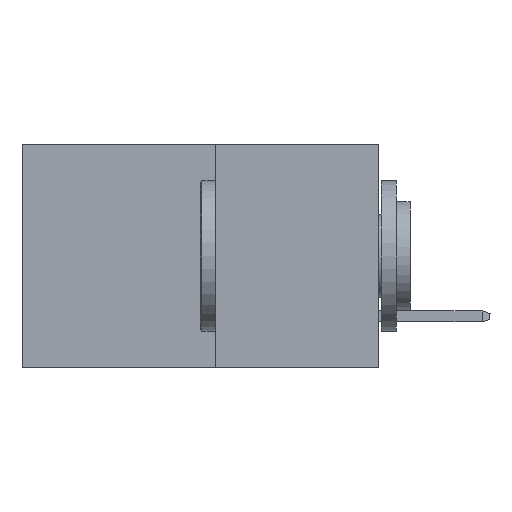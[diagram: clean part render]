
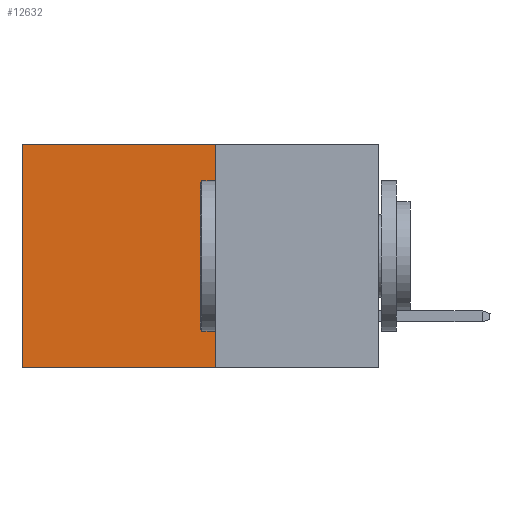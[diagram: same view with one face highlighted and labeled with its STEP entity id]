
A CAD part, left-side view. The second image highlights one B-rep face of the part: STEP entity #12632.
In plain terms, the highlighted planar face has unit normal (-1, 0, 0).
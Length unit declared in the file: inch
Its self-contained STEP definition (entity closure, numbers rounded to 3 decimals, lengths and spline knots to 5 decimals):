
#191 = EDGE_CURVE ( 'NONE', #2606, #7207, #2613, .T. ) ;
#749 = VECTOR ( 'NONE', #18762, 39.37008 ) ;
#1386 = ORIENTED_EDGE ( 'NONE', *, *, #4446, .T. ) ;
#1674 = VERTEX_POINT ( 'NONE', #5386 ) ;
#2606 = VERTEX_POINT ( 'NONE', #9807 ) ;
#2611 = CARTESIAN_POINT ( 'NONE',  ( 0.277, 0.27, 0. ) ) ;
#2613 = LINE ( 'NONE', #2611, #6604 ) ;
#3607 = ORIENTED_EDGE ( 'NONE', *, *, #17054, .F. ) ;
#4293 = PLANE ( 'NONE',  #8419 ) ;
#4446 = EDGE_CURVE ( 'NONE', #7207, #8948, #5085, .T. ) ;
#4540 = VECTOR ( 'NONE', #20747, 39.37008 ) ;
#5085 = LINE ( 'NONE', #20797, #4540 ) ;
#5386 = CARTESIAN_POINT ( 'NONE',  ( 0.277, 0.27, -0.37 ) ) ;
#5595 = CARTESIAN_POINT ( 'NONE',  ( 0.277, 0.27, -0.37 ) ) ;
#6604 = VECTOR ( 'NONE', #13789, 39.37008 ) ;
#7207 = VERTEX_POINT ( 'NONE', #15100 ) ;
#7413 = ORIENTED_EDGE ( 'NONE', *, *, #19953, .F. ) ;
#7571 = CARTESIAN_POINT ( 'NONE',  ( 0.277, 0.27, -0.37 ) ) ;
#7633 = FACE_OUTER_BOUND ( 'NONE', #19626, .T. ) ;
#7637 = DIRECTION ( 'NONE',  ( 0., 0., -1. ) ) ;
#8419 = AXIS2_PLACEMENT_3D ( 'NONE', #7571, #17523, #7637 ) ;
#8663 = VECTOR ( 'NONE', #21054, 39.37008 ) ;
#8948 = VERTEX_POINT ( 'NONE', #12015 ) ;
#9196 = LINE ( 'NONE', #19438, #8663 ) ;
#9677 = LINE ( 'NONE', #5595, #749 ) ;
#9807 = CARTESIAN_POINT ( 'NONE',  ( 0.277, 0.27, 0. ) ) ;
#12015 = CARTESIAN_POINT ( 'NONE',  ( 0.277, 0.59, -0.37 ) ) ;
#12632 = ADVANCED_FACE ( 'NONE', ( #7633 ), #4293, .F. ) ;
#13789 = DIRECTION ( 'NONE',  ( 0., 1., 0. ) ) ;
#15100 = CARTESIAN_POINT ( 'NONE',  ( 0.277, 0.59, 0. ) ) ;
#15321 = ORIENTED_EDGE ( 'NONE', *, *, #191, .T. ) ;
#17054 = EDGE_CURVE ( 'NONE', #1674, #8948, #9677, .T. ) ;
#17523 = DIRECTION ( 'NONE',  ( 1., 0., 0. ) ) ;
#18762 = DIRECTION ( 'NONE',  ( 0., 1., 0. ) ) ;
#19438 = CARTESIAN_POINT ( 'NONE',  ( 0.277, 0.27, -0.37 ) ) ;
#19626 = EDGE_LOOP ( 'NONE', ( #1386, #3607, #7413, #15321 ) ) ;
#19953 = EDGE_CURVE ( 'NONE', #2606, #1674, #9196, .T. ) ;
#20747 = DIRECTION ( 'NONE',  ( 0., 0., -1. ) ) ;
#20797 = CARTESIAN_POINT ( 'NONE',  ( 0.277, 0.59, -0.37 ) ) ;
#21054 = DIRECTION ( 'NONE',  ( 0., 0., -1. ) ) ;
